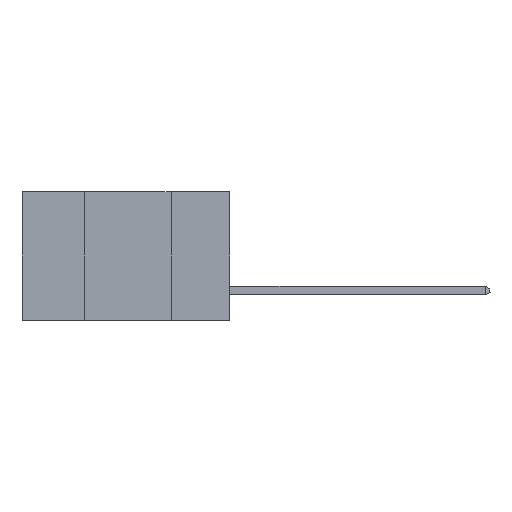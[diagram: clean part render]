
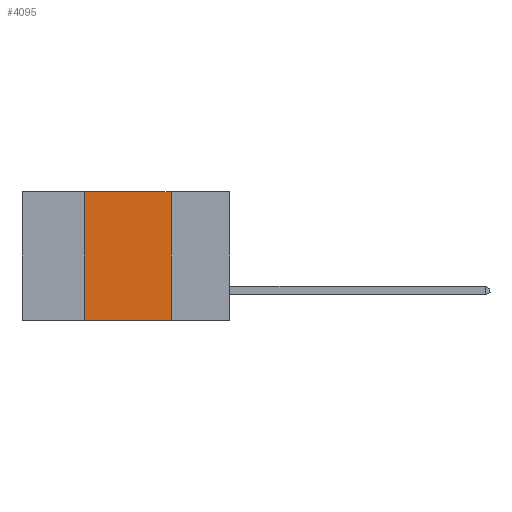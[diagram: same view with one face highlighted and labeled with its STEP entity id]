
A CAD part, left-side view. The second image highlights one B-rep face of the part: STEP entity #4095.
In plain terms, the highlighted planar face has unit normal (-1, 0, 0).
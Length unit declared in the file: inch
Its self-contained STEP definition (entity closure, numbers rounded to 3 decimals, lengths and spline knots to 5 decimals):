
#395 = VERTEX_POINT ( 'NONE', #14411 ) ;
#808 = EDGE_LOOP ( 'NONE', ( #2032, #18660, #19735, #19259 ) ) ;
#910 = VECTOR ( 'NONE', #5437, 39.37008 ) ;
#950 = DIRECTION ( 'NONE',  ( 0., 0., 1. ) ) ;
#1005 = VERTEX_POINT ( 'NONE', #18542 ) ;
#2032 = ORIENTED_EDGE ( 'NONE', *, *, #4248, .F. ) ;
#2107 = LINE ( 'NONE', #3259, #18647 ) ;
#3259 = CARTESIAN_POINT ( 'NONE',  ( 0., 0.6, 0. ) ) ;
#3261 = CARTESIAN_POINT ( 'NONE',  ( 0., 0.6, 0. ) ) ;
#4023 = EDGE_CURVE ( 'NONE', #6346, #395, #18655, .T. ) ;
#4062 = CARTESIAN_POINT ( 'NONE',  ( 0., 0.42, 0. ) ) ;
#4095 = ADVANCED_FACE ( 'NONE', ( #15142 ), #10654, .F. ) ;
#4248 = EDGE_CURVE ( 'NONE', #7282, #395, #11975, .T. ) ;
#4552 = DIRECTION ( 'NONE',  ( 1., 0., 0. ) ) ;
#4560 = AXIS2_PLACEMENT_3D ( 'NONE', #3261, #4552, #12418 ) ;
#5437 = DIRECTION ( 'NONE',  ( 0., -1., 0. ) ) ;
#6346 = VERTEX_POINT ( 'NONE', #14147 ) ;
#6447 = CARTESIAN_POINT ( 'NONE',  ( 0., 0.17, 0. ) ) ;
#6463 = LINE ( 'NONE', #4062, #18406 ) ;
#6815 = CARTESIAN_POINT ( 'NONE',  ( 0., 0.17, 0. ) ) ;
#7211 = CARTESIAN_POINT ( 'NONE',  ( 0., 0.6, -0.37 ) ) ;
#7282 = VERTEX_POINT ( 'NONE', #6815 ) ;
#8820 = VECTOR ( 'NONE', #17324, 39.37008 ) ;
#9494 = DIRECTION ( 'NONE',  ( 0., -1., 0. ) ) ;
#9638 = EDGE_CURVE ( 'NONE', #1005, #7282, #2107, .T. ) ;
#10654 = PLANE ( 'NONE',  #4560 ) ;
#11975 = LINE ( 'NONE', #6447, #8820 ) ;
#12418 = DIRECTION ( 'NONE',  ( 0., 0., -1. ) ) ;
#14147 = CARTESIAN_POINT ( 'NONE',  ( 0., 0.42, -0.37 ) ) ;
#14411 = CARTESIAN_POINT ( 'NONE',  ( 0., 0.17, -0.37 ) ) ;
#15142 = FACE_OUTER_BOUND ( 'NONE', #808, .T. ) ;
#16815 = EDGE_CURVE ( 'NONE', #6346, #1005, #6463, .T. ) ;
#17324 = DIRECTION ( 'NONE',  ( 0., 0., -1. ) ) ;
#18406 = VECTOR ( 'NONE', #950, 39.37008 ) ;
#18542 = CARTESIAN_POINT ( 'NONE',  ( 0., 0.42, 0. ) ) ;
#18647 = VECTOR ( 'NONE', #9494, 39.37008 ) ;
#18655 = LINE ( 'NONE', #7211, #910 ) ;
#18660 = ORIENTED_EDGE ( 'NONE', *, *, #9638, .F. ) ;
#19259 = ORIENTED_EDGE ( 'NONE', *, *, #4023, .T. ) ;
#19735 = ORIENTED_EDGE ( 'NONE', *, *, #16815, .F. ) ;
